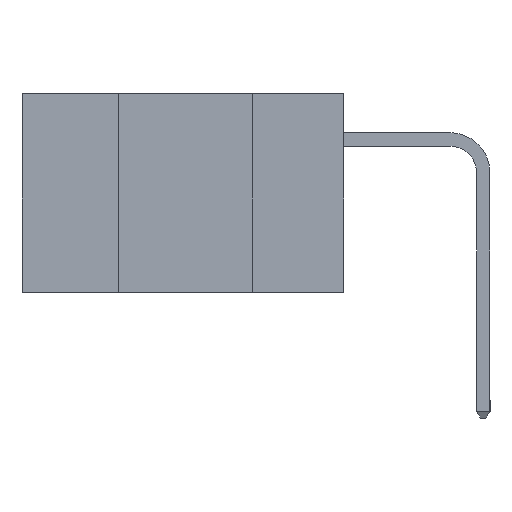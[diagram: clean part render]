
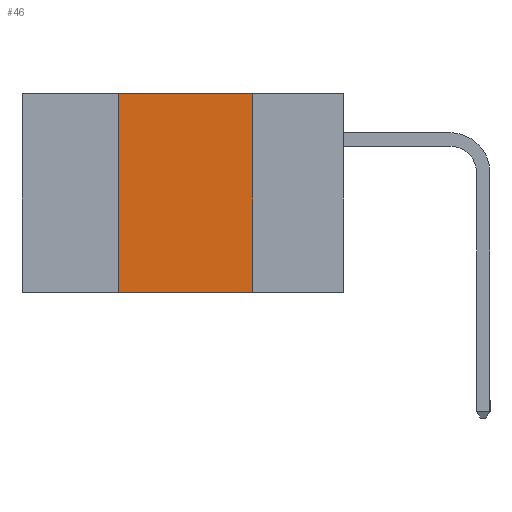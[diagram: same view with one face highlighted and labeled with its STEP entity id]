
A CAD part, left-side view. The second image highlights one B-rep face of the part: STEP entity #46.
In plain terms, the highlighted planar face has unit normal (-1, 0, 0).
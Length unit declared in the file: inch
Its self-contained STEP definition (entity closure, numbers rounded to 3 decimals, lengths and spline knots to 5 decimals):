
#46 = ADVANCED_FACE ( 'NONE', ( #8240 ), #880, .F. ) ;
#880 = PLANE ( 'NONE',  #9709 ) ;
#1140 = DIRECTION ( 'NONE',  ( 0., -1., 0. ) ) ;
#1411 = EDGE_CURVE ( 'NONE', #4145, #5785, #2484, .T. ) ;
#1415 = ORIENTED_EDGE ( 'NONE', *, *, #1411, .F. ) ;
#1687 = EDGE_CURVE ( 'NONE', #5785, #2757, #8513, .T. ) ;
#1887 = ORIENTED_EDGE ( 'NONE', *, *, #1687, .F. ) ;
#1937 = DIRECTION ( 'NONE',  ( 0., 0., -1. ) ) ;
#2484 = LINE ( 'NONE', #5075, #10626 ) ;
#2716 = ORIENTED_EDGE ( 'NONE', *, *, #12522, .F. ) ;
#2757 = VERTEX_POINT ( 'NONE', #8855 ) ;
#3542 = EDGE_CURVE ( 'NONE', #4145, #10725, #9870, .T. ) ;
#3555 = DIRECTION ( 'NONE',  ( 0., 0., -1. ) ) ;
#4145 = VERTEX_POINT ( 'NONE', #6532 ) ;
#4331 = CARTESIAN_POINT ( 'NONE',  ( 0., 0.6, -0.37 ) ) ;
#5075 = CARTESIAN_POINT ( 'NONE',  ( 0., 0.42, -0.37 ) ) ;
#5224 = CARTESIAN_POINT ( 'NONE',  ( 0., 0.6, 0. ) ) ;
#5276 = LINE ( 'NONE', #11301, #13807 ) ;
#5785 = VERTEX_POINT ( 'NONE', #6534 ) ;
#5993 = CARTESIAN_POINT ( 'NONE',  ( 0., 0.17, -0.37 ) ) ;
#6184 = DIRECTION ( 'NONE',  ( 0., 0., 1. ) ) ;
#6532 = CARTESIAN_POINT ( 'NONE',  ( 0., 0.42, -0.37 ) ) ;
#6534 = CARTESIAN_POINT ( 'NONE',  ( 0., 0.42, 0. ) ) ;
#6592 = ORIENTED_EDGE ( 'NONE', *, *, #3542, .T. ) ;
#6855 = EDGE_LOOP ( 'NONE', ( #2716, #1887, #1415, #6592 ) ) ;
#7854 = DIRECTION ( 'NONE',  ( 0., -1., 0. ) ) ;
#8240 = FACE_OUTER_BOUND ( 'NONE', #6855, .T. ) ;
#8513 = LINE ( 'NONE', #10048, #12857 ) ;
#8855 = CARTESIAN_POINT ( 'NONE',  ( 0., 0.17, 0. ) ) ;
#9709 = AXIS2_PLACEMENT_3D ( 'NONE', #5224, #14208, #1937 ) ;
#9870 = LINE ( 'NONE', #4331, #12120 ) ;
#10048 = CARTESIAN_POINT ( 'NONE',  ( 0., 0.6, 0. ) ) ;
#10626 = VECTOR ( 'NONE', #6184, 39.37008 ) ;
#10725 = VERTEX_POINT ( 'NONE', #5993 ) ;
#11301 = CARTESIAN_POINT ( 'NONE',  ( 0., 0.17, -0.37 ) ) ;
#12120 = VECTOR ( 'NONE', #1140, 39.37008 ) ;
#12522 = EDGE_CURVE ( 'NONE', #2757, #10725, #5276, .T. ) ;
#12857 = VECTOR ( 'NONE', #7854, 39.37008 ) ;
#13807 = VECTOR ( 'NONE', #3555, 39.37008 ) ;
#14208 = DIRECTION ( 'NONE',  ( 1., 0., 0. ) ) ;
